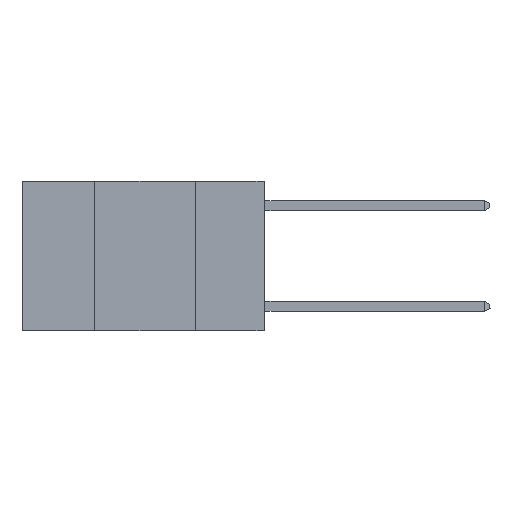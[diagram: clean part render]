
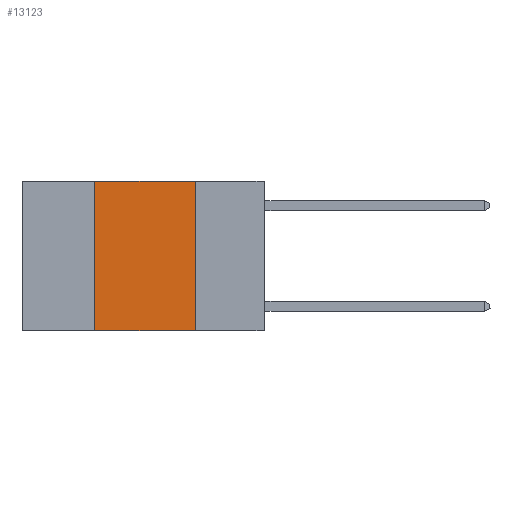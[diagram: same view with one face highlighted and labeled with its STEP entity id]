
A CAD part, left-side view. The second image highlights one B-rep face of the part: STEP entity #13123.
In plain terms, the highlighted planar face has unit normal (-1, 0, 0).
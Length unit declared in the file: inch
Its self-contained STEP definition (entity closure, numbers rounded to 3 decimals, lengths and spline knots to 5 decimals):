
#790 = VERTEX_POINT ( 'NONE', #949 ) ;
#949 = CARTESIAN_POINT ( 'NONE',  ( 0., 0.42, 0. ) ) ;
#1594 = LINE ( 'NONE', #11926, #7291 ) ;
#1861 = DIRECTION ( 'NONE',  ( 0., -1., 0. ) ) ;
#4008 = PLANE ( 'NONE',  #16954 ) ;
#4959 = LINE ( 'NONE', #9253, #18570 ) ;
#5090 = EDGE_CURVE ( 'NONE', #13765, #22417, #4959, .T. ) ;
#7291 = VECTOR ( 'NONE', #1861, 39.37008 ) ;
#7719 = CARTESIAN_POINT ( 'NONE',  ( 0., 0.42, -0.37 ) ) ;
#8135 = EDGE_CURVE ( 'NONE', #13367, #790, #15846, .T. ) ;
#8279 = LINE ( 'NONE', #12114, #20369 ) ;
#9253 = CARTESIAN_POINT ( 'NONE',  ( 0., 0.17, 0. ) ) ;
#9605 = ORIENTED_EDGE ( 'NONE', *, *, #21860, .F. ) ;
#11926 = CARTESIAN_POINT ( 'NONE',  ( 0., 0.6, 0. ) ) ;
#12114 = CARTESIAN_POINT ( 'NONE',  ( 0., 0.6, -0.37 ) ) ;
#12131 = ORIENTED_EDGE ( 'NONE', *, *, #8135, .F. ) ;
#12420 = DIRECTION ( 'NONE',  ( 1., 0., 0. ) ) ;
#13123 = ADVANCED_FACE ( 'NONE', ( #14499 ), #4008, .F. ) ;
#13367 = VERTEX_POINT ( 'NONE', #7719 ) ;
#13765 = VERTEX_POINT ( 'NONE', #20734 ) ;
#13927 = DIRECTION ( 'NONE',  ( 0., 0., 1. ) ) ;
#14345 = ORIENTED_EDGE ( 'NONE', *, *, #16524, .T. ) ;
#14499 = FACE_OUTER_BOUND ( 'NONE', #17694, .T. ) ;
#15846 = LINE ( 'NONE', #24390, #19020 ) ;
#16524 = EDGE_CURVE ( 'NONE', #13367, #22417, #8279, .T. ) ;
#16671 = DIRECTION ( 'NONE',  ( 0., -1., 0. ) ) ;
#16954 = AXIS2_PLACEMENT_3D ( 'NONE', #22889, #12420, #20834 ) ;
#17642 = DIRECTION ( 'NONE',  ( 0., 0., -1. ) ) ;
#17694 = EDGE_LOOP ( 'NONE', ( #18311, #9605, #12131, #14345 ) ) ;
#18311 = ORIENTED_EDGE ( 'NONE', *, *, #5090, .F. ) ;
#18570 = VECTOR ( 'NONE', #17642, 39.37008 ) ;
#19020 = VECTOR ( 'NONE', #13927, 39.37008 ) ;
#19731 = CARTESIAN_POINT ( 'NONE',  ( 0., 0.17, -0.37 ) ) ;
#20369 = VECTOR ( 'NONE', #16671, 39.37008 ) ;
#20734 = CARTESIAN_POINT ( 'NONE',  ( 0., 0.17, 0. ) ) ;
#20834 = DIRECTION ( 'NONE',  ( 0., 0., -1. ) ) ;
#21860 = EDGE_CURVE ( 'NONE', #790, #13765, #1594, .T. ) ;
#22417 = VERTEX_POINT ( 'NONE', #19731 ) ;
#22889 = CARTESIAN_POINT ( 'NONE',  ( 0., 0.6, 0. ) ) ;
#24390 = CARTESIAN_POINT ( 'NONE',  ( 0., 0.42, 0. ) ) ;
